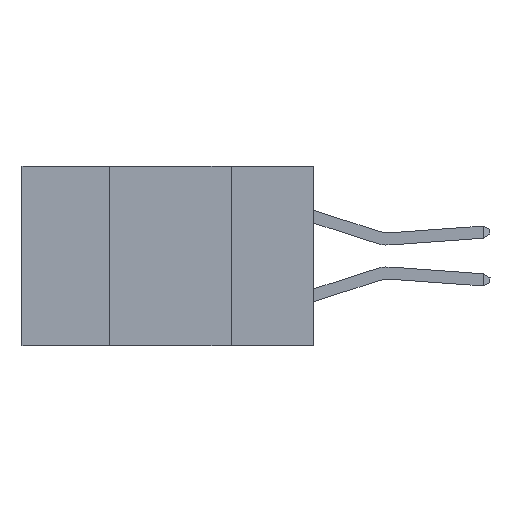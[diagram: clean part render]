
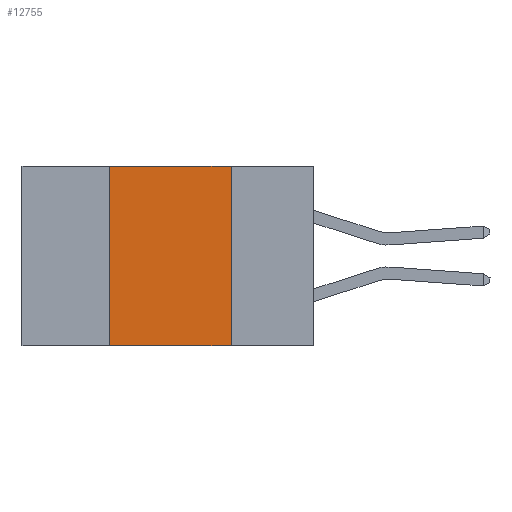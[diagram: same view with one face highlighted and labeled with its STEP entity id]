
A CAD part, left-side view. The second image highlights one B-rep face of the part: STEP entity #12755.
In plain terms, the highlighted planar face has unit normal (-1, 0, 0).
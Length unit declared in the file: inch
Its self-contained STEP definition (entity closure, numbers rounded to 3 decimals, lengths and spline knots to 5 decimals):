
#120 = VERTEX_POINT ( 'NONE', #7985 ) ;
#411 = LINE ( 'NONE', #15722, #12100 ) ;
#1808 = CARTESIAN_POINT ( 'NONE',  ( 0., 0.6, -0.37 ) ) ;
#1892 = VERTEX_POINT ( 'NONE', #16363 ) ;
#2734 = DIRECTION ( 'NONE',  ( 0., 0., -1. ) ) ;
#2886 = LINE ( 'NONE', #12034, #13923 ) ;
#2954 = VERTEX_POINT ( 'NONE', #13067 ) ;
#2999 = ORIENTED_EDGE ( 'NONE', *, *, #18641, .F. ) ;
#3646 = ORIENTED_EDGE ( 'NONE', *, *, #13652, .F. ) ;
#4492 = VECTOR ( 'NONE', #14919, 39.37008 ) ;
#4825 = DIRECTION ( 'NONE',  ( 0., -1., 0. ) ) ;
#6032 = EDGE_CURVE ( 'NONE', #120, #1892, #411, .T. ) ;
#6891 = VECTOR ( 'NONE', #4825, 39.37008 ) ;
#6958 = EDGE_CURVE ( 'NONE', #2954, #1892, #7801, .T. ) ;
#7176 = DIRECTION ( 'NONE',  ( 0., 0., -1. ) ) ;
#7773 = ORIENTED_EDGE ( 'NONE', *, *, #6958, .T. ) ;
#7801 = LINE ( 'NONE', #1808, #6891 ) ;
#7985 = CARTESIAN_POINT ( 'NONE',  ( 0., 0.17, 0. ) ) ;
#9796 = LINE ( 'NONE', #16457, #4492 ) ;
#10009 = CARTESIAN_POINT ( 'NONE',  ( 0., 0.6, 0. ) ) ;
#12034 = CARTESIAN_POINT ( 'NONE',  ( 0., 0.6, 0. ) ) ;
#12100 = VECTOR ( 'NONE', #2734, 39.37008 ) ;
#12755 = ADVANCED_FACE ( 'NONE', ( #18282 ), #12864, .F. ) ;
#12864 = PLANE ( 'NONE',  #15346 ) ;
#13067 = CARTESIAN_POINT ( 'NONE',  ( 0., 0.42, -0.37 ) ) ;
#13652 = EDGE_CURVE ( 'NONE', #2954, #18220, #9796, .T. ) ;
#13923 = VECTOR ( 'NONE', #17695, 39.37008 ) ;
#14482 = ORIENTED_EDGE ( 'NONE', *, *, #6032, .F. ) ;
#14919 = DIRECTION ( 'NONE',  ( 0., 0., 1. ) ) ;
#15346 = AXIS2_PLACEMENT_3D ( 'NONE', #10009, #15730, #7176 ) ;
#15722 = CARTESIAN_POINT ( 'NONE',  ( 0., 0.17, 0. ) ) ;
#15730 = DIRECTION ( 'NONE',  ( 1., 0., 0. ) ) ;
#16363 = CARTESIAN_POINT ( 'NONE',  ( 0., 0.17, -0.37 ) ) ;
#16457 = CARTESIAN_POINT ( 'NONE',  ( 0., 0.42, 0. ) ) ;
#16836 = CARTESIAN_POINT ( 'NONE',  ( 0., 0.42, 0. ) ) ;
#17216 = EDGE_LOOP ( 'NONE', ( #14482, #2999, #3646, #7773 ) ) ;
#17695 = DIRECTION ( 'NONE',  ( 0., -1., 0. ) ) ;
#18220 = VERTEX_POINT ( 'NONE', #16836 ) ;
#18282 = FACE_OUTER_BOUND ( 'NONE', #17216, .T. ) ;
#18641 = EDGE_CURVE ( 'NONE', #18220, #120, #2886, .T. ) ;
